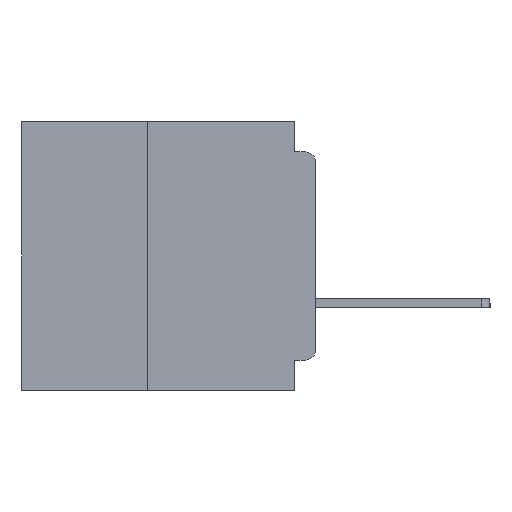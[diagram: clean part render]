
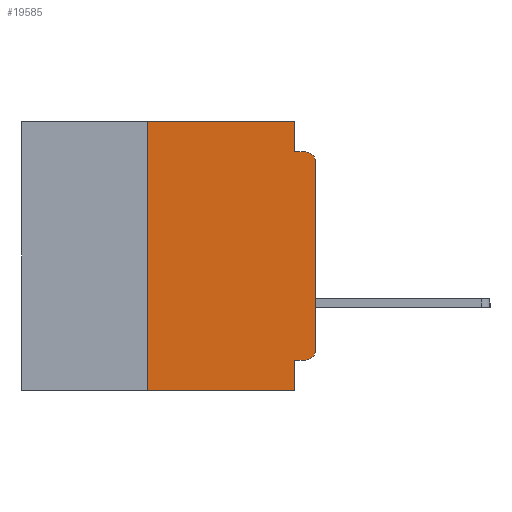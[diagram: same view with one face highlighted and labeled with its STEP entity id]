
A CAD part, left-side view. The second image highlights one B-rep face of the part: STEP entity #19585.
In plain terms, the highlighted planar face has unit normal (-1, 0, 0).
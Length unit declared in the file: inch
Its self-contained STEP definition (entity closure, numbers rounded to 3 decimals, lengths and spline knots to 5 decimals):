
#110 = CARTESIAN_POINT ( 'NONE',  ( 0., 0.437, -0.4 ) ) ;
#2065 = CARTESIAN_POINT ( 'NONE',  ( 0., 0.437, 0. ) ) ;
#2296 = VERTEX_POINT ( 'NONE', #31972 ) ;
#2576 = ORIENTED_EDGE ( 'NONE', *, *, #34540, .T. ) ;
#3163 = CARTESIAN_POINT ( 'NONE',  ( 0., 0.25, -0.4 ) ) ;
#4217 = CARTESIAN_POINT ( 'NONE',  ( 0., 0.015, -0.34 ) ) ;
#4997 = CARTESIAN_POINT ( 'NONE',  ( 0., 0., -0.06 ) ) ;
#5499 = CARTESIAN_POINT ( 'NONE',  ( 0., 0.031, 0. ) ) ;
#6342 = LINE ( 'NONE', #7869, #38170 ) ;
#6486 = ORIENTED_EDGE ( 'NONE', *, *, #31685, .T. ) ;
#7300 = CARTESIAN_POINT ( 'NONE',  ( 0., 0.031, -0.045 ) ) ;
#7376 = DIRECTION ( 'NONE',  ( 0., 0., -1. ) ) ;
#7472 = VECTOR ( 'NONE', #25015, 39.37008 ) ;
#7869 = CARTESIAN_POINT ( 'NONE',  ( 0., 0., -0.355 ) ) ;
#8005 = VECTOR ( 'NONE', #11508, 39.37008 ) ;
#8022 = EDGE_CURVE ( 'NONE', #40028, #37861, #22934, .T. ) ;
#8256 = VECTOR ( 'NONE', #18999, 39.37008 ) ;
#8274 = EDGE_CURVE ( 'NONE', #33436, #40028, #22444, .T. ) ;
#8318 = EDGE_CURVE ( 'NONE', #15049, #21778, #31559, .T. ) ;
#9359 = EDGE_CURVE ( 'NONE', #37861, #37610, #16556, .T. ) ;
#11040 = DIRECTION ( 'NONE',  ( 0., 1., 0. ) ) ;
#11508 = DIRECTION ( 'NONE',  ( 0., 0., 1. ) ) ;
#11637 = CIRCLE ( 'NONE', #21665, 0.015 ) ;
#11683 = ORIENTED_EDGE ( 'NONE', *, *, #8022, .F. ) ;
#12360 = AXIS2_PLACEMENT_3D ( 'NONE', #34603, #16200, #37638 ) ;
#12622 = ORIENTED_EDGE ( 'NONE', *, *, #9359, .F. ) ;
#12797 = AXIS2_PLACEMENT_3D ( 'NONE', #4217, #25914, #7376 ) ;
#12976 = CARTESIAN_POINT ( 'NONE',  ( 0., 0.015, -0.355 ) ) ;
#13357 = CIRCLE ( 'NONE', #12797, 0.015 ) ;
#13602 = ORIENTED_EDGE ( 'NONE', *, *, #8274, .F. ) ;
#13882 = VERTEX_POINT ( 'NONE', #4997 ) ;
#15049 = VERTEX_POINT ( 'NONE', #16587 ) ;
#15873 = CARTESIAN_POINT ( 'NONE',  ( 0., 0.031, 0. ) ) ;
#15887 = DIRECTION ( 'NONE',  ( 0., 0., -1. ) ) ;
#16200 = DIRECTION ( 'NONE',  ( 1., 0., 0. ) ) ;
#16218 = ORIENTED_EDGE ( 'NONE', *, *, #26299, .T. ) ;
#16556 = LINE ( 'NONE', #15873, #8256 ) ;
#16587 = CARTESIAN_POINT ( 'NONE',  ( 0., 0.031, -0.355 ) ) ;
#17578 = CARTESIAN_POINT ( 'NONE',  ( 0., 0.015, -0.06 ) ) ;
#18999 = DIRECTION ( 'NONE',  ( 0., 0., -1. ) ) ;
#19219 = CARTESIAN_POINT ( 'NONE',  ( 0., 0.031, -0.4 ) ) ;
#19585 = ADVANCED_FACE ( 'NONE', ( #19708 ), #28417, .F. ) ;
#19665 = EDGE_LOOP ( 'NONE', ( #16218, #2576, #27341, #12622, #11683, #13602, #21809, #39070, #33518, #6486 ) ) ;
#19708 = FACE_OUTER_BOUND ( 'NONE', #19665, .T. ) ;
#19900 = CARTESIAN_POINT ( 'NONE',  ( 0., 0.25, -0.4 ) ) ;
#20075 = EDGE_CURVE ( 'NONE', #33436, #21778, #22998, .T. ) ;
#20511 = VECTOR ( 'NONE', #15887, 39.37008 ) ;
#20681 = DIRECTION ( 'NONE',  ( 0., 0., -1. ) ) ;
#20755 = DIRECTION ( 'NONE',  ( 0., -1., 0. ) ) ;
#21220 = CARTESIAN_POINT ( 'NONE',  ( 0., 0., -0.34 ) ) ;
#21580 = VERTEX_POINT ( 'NONE', #21220 ) ;
#21665 = AXIS2_PLACEMENT_3D ( 'NONE', #17578, #39016, #20681 ) ;
#21778 = VERTEX_POINT ( 'NONE', #19219 ) ;
#21809 = ORIENTED_EDGE ( 'NONE', *, *, #20075, .T. ) ;
#22095 = CARTESIAN_POINT ( 'NONE',  ( 0., 0.031, -0.4 ) ) ;
#22444 = LINE ( 'NONE', #3163, #37752 ) ;
#22934 = LINE ( 'NONE', #2065, #31090 ) ;
#22998 = LINE ( 'NONE', #110, #7472 ) ;
#23212 = VERTEX_POINT ( 'NONE', #12976 ) ;
#24902 = DIRECTION ( 'NONE',  ( 0., 0., 1. ) ) ;
#25015 = DIRECTION ( 'NONE',  ( 0., -1., 0. ) ) ;
#25651 = VECTOR ( 'NONE', #39472, 39.37008 ) ;
#25914 = DIRECTION ( 'NONE',  ( -1., 0., 0. ) ) ;
#26299 = EDGE_CURVE ( 'NONE', #21580, #13882, #31689, .T. ) ;
#26612 = LINE ( 'NONE', #30273, #25651 ) ;
#27341 = ORIENTED_EDGE ( 'NONE', *, *, #34356, .F. ) ;
#28417 = PLANE ( 'NONE',  #12360 ) ;
#29956 = CARTESIAN_POINT ( 'NONE',  ( 0., 0., 0. ) ) ;
#30273 = CARTESIAN_POINT ( 'NONE',  ( 0., 0., -0.045 ) ) ;
#31090 = VECTOR ( 'NONE', #20755, 39.37008 ) ;
#31559 = LINE ( 'NONE', #22095, #20511 ) ;
#31685 = EDGE_CURVE ( 'NONE', #23212, #21580, #13357, .T. ) ;
#31689 = LINE ( 'NONE', #29956, #8005 ) ;
#31972 = CARTESIAN_POINT ( 'NONE',  ( 0., 0.015, -0.045 ) ) ;
#33436 = VERTEX_POINT ( 'NONE', #19900 ) ;
#33518 = ORIENTED_EDGE ( 'NONE', *, *, #37197, .F. ) ;
#34356 = EDGE_CURVE ( 'NONE', #37610, #2296, #26612, .T. ) ;
#34540 = EDGE_CURVE ( 'NONE', #13882, #2296, #11637, .T. ) ;
#34603 = CARTESIAN_POINT ( 'NONE',  ( 0., 0.437, 0. ) ) ;
#37197 = EDGE_CURVE ( 'NONE', #23212, #15049, #6342, .T. ) ;
#37610 = VERTEX_POINT ( 'NONE', #7300 ) ;
#37638 = DIRECTION ( 'NONE',  ( 0., 0., -1. ) ) ;
#37752 = VECTOR ( 'NONE', #24902, 39.37008 ) ;
#37861 = VERTEX_POINT ( 'NONE', #5499 ) ;
#38170 = VECTOR ( 'NONE', #11040, 39.37008 ) ;
#39016 = DIRECTION ( 'NONE',  ( -1., 0., 0. ) ) ;
#39070 = ORIENTED_EDGE ( 'NONE', *, *, #8318, .F. ) ;
#39472 = DIRECTION ( 'NONE',  ( 0., -1., 0. ) ) ;
#39586 = CARTESIAN_POINT ( 'NONE',  ( 0., 0.25, 0. ) ) ;
#40028 = VERTEX_POINT ( 'NONE', #39586 ) ;
